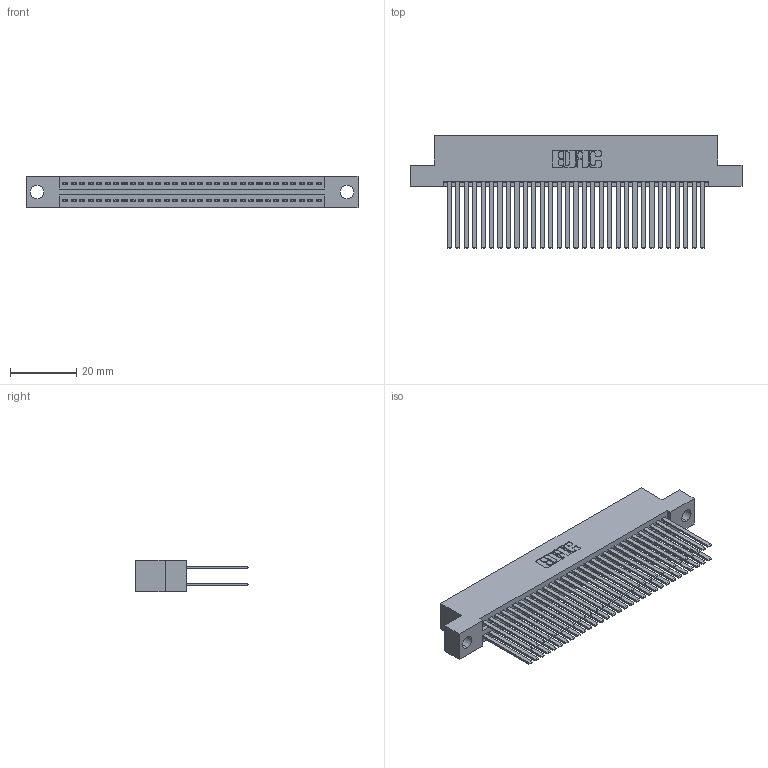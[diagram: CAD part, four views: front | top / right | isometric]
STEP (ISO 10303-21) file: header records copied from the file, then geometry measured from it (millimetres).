
FILE_DESCRIPTION (( 'STEP AP203' ), '1' );
FILE_NAME ('395-062-544-204.STEP', '2021-06-17T02:35:38', ( '' ), ( '' ), 'SwSTEP 2.0', 'SolidWorks 2020', '' );
FILE_SCHEMA (( 'CONFIG_CONTROL_DESIGN' ));
Length unit declared in the file: inch
Products named in the file (3): 345 Part_Flush Mounting Lugs - 0.156 Dia-TI; 395-062-544-204; 345-292-001_345-293-144
Assembly tree (63 placements, depth 2):
  395-062-544-204
    345 Part_Flush Mounting Lugs - 0.156 Dia-TI
    345-292-001_345-293-144  x62
Bounding box: 99.95 x 33.96 x 9.4 mm (x, y, z)
Volume: 10370.2 mm3; surface area: 17514.8 mm2
Topology: 63 solids, 63 shells, 2868 faces, 8499 edges, 5582 vertices
Faces by surface type: plane 1892, cylinder 976
Entity records: 26039 total; most frequent: CARTESIAN_POINT 4378, ORIENTED_EDGE 4310, DIRECTION 3871, EDGE_CURVE 2155, VECTOR 1903, LINE 1903, VERTEX_POINT 1434, AXIS2_PLACEMENT_3D 984
